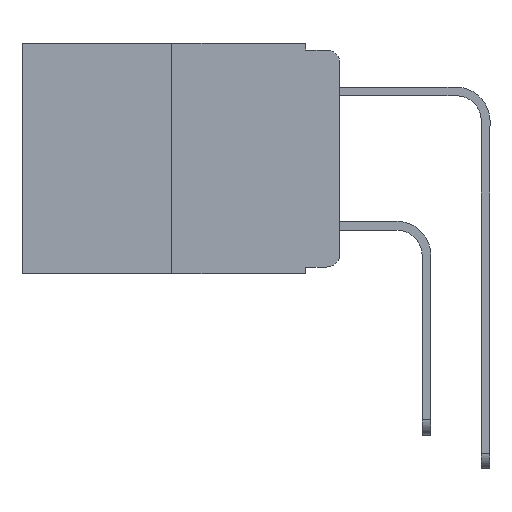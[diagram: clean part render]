
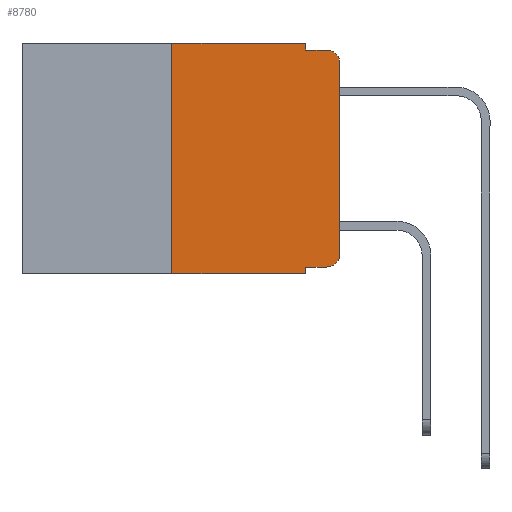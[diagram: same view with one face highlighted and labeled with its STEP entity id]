
A CAD part, left-side view. The second image highlights one B-rep face of the part: STEP entity #8780.
In plain terms, the highlighted planar face has unit normal (-1, 0, 0).
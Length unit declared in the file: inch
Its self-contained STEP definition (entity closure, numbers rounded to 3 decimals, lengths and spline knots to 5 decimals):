
#59 = VERTEX_POINT ( 'NONE', #3711 ) ;
#158 = VECTOR ( 'NONE', #4470, 39.37008 ) ;
#255 = DIRECTION ( 'NONE',  ( 0., 0., -1. ) ) ;
#367 = DIRECTION ( 'NONE',  ( 0., 0., -1. ) ) ;
#1039 = CARTESIAN_POINT ( 'NONE',  ( 0., 0.051, -0.01 ) ) ;
#1134 = LINE ( 'NONE', #12113, #1515 ) ;
#1308 = LINE ( 'NONE', #9074, #10703 ) ;
#1515 = VECTOR ( 'NONE', #367, 39.37008 ) ;
#1615 = LINE ( 'NONE', #4549, #13292 ) ;
#1960 = DIRECTION ( 'NONE',  ( 0., 0., 1. ) ) ;
#2012 = DIRECTION ( 'NONE',  ( -1., 0., 0. ) ) ;
#2083 = VERTEX_POINT ( 'NONE', #13262 ) ;
#2281 = DIRECTION ( 'NONE',  ( 0., -1., 0. ) ) ;
#2284 = LINE ( 'NONE', #9233, #8231 ) ;
#2569 = ORIENTED_EDGE ( 'NONE', *, *, #5013, .T. ) ;
#2573 = CARTESIAN_POINT ( 'NONE',  ( 0., 0.473, 0. ) ) ;
#3114 = ORIENTED_EDGE ( 'NONE', *, *, #7269, .F. ) ;
#3270 = VECTOR ( 'NONE', #5483, 39.37008 ) ;
#3467 = VECTOR ( 'NONE', #14346, 39.37008 ) ;
#3666 = ORIENTED_EDGE ( 'NONE', *, *, #6000, .F. ) ;
#3711 = CARTESIAN_POINT ( 'NONE',  ( 0., 0.25, -0.343 ) ) ;
#3911 = AXIS2_PLACEMENT_3D ( 'NONE', #9136, #2012, #10263 ) ;
#4214 = ORIENTED_EDGE ( 'NONE', *, *, #4797, .F. ) ;
#4291 = CARTESIAN_POINT ( 'NONE',  ( 0., 0.25, 0. ) ) ;
#4322 = CARTESIAN_POINT ( 'NONE',  ( 0., 0.02, -0.03 ) ) ;
#4470 = DIRECTION ( 'NONE',  ( 0., -1., 0. ) ) ;
#4549 = CARTESIAN_POINT ( 'NONE',  ( 0., 0.051, -0.333 ) ) ;
#4797 = EDGE_CURVE ( 'NONE', #13849, #8151, #1134, .T. ) ;
#4871 = CARTESIAN_POINT ( 'NONE',  ( 0., 0., -0.03 ) ) ;
#4902 = PLANE ( 'NONE',  #8077 ) ;
#5013 = EDGE_CURVE ( 'NONE', #2083, #12162, #1308, .T. ) ;
#5483 = DIRECTION ( 'NONE',  ( 0., 0., 1. ) ) ;
#5524 = DIRECTION ( 'NONE',  ( 0., 0., -1. ) ) ;
#6000 = EDGE_CURVE ( 'NONE', #6590, #13849, #9615, .T. ) ;
#6093 = LINE ( 'NONE', #12098, #3467 ) ;
#6144 = CARTESIAN_POINT ( 'NONE',  ( 0., 0.02, -0.01 ) ) ;
#6302 = ORIENTED_EDGE ( 'NONE', *, *, #8257, .T. ) ;
#6590 = VERTEX_POINT ( 'NONE', #6793 ) ;
#6793 = CARTESIAN_POINT ( 'NONE',  ( 0., 0.25, 0. ) ) ;
#6828 = EDGE_LOOP ( 'NONE', ( #2569, #6302, #3114, #4214, #3666, #13722, #14591, #10012, #12701, #13752 ) ) ;
#7088 = CARTESIAN_POINT ( 'NONE',  ( 0., 0.051, -0.333 ) ) ;
#7269 = EDGE_CURVE ( 'NONE', #8151, #12727, #9402, .T. ) ;
#7300 = EDGE_CURVE ( 'NONE', #7944, #7658, #1615, .T. ) ;
#7374 = DIRECTION ( 'NONE',  ( 1., 0., 0. ) ) ;
#7658 = VERTEX_POINT ( 'NONE', #10017 ) ;
#7944 = VERTEX_POINT ( 'NONE', #7088 ) ;
#8077 = AXIS2_PLACEMENT_3D ( 'NONE', #2573, #7374, #255 ) ;
#8148 = DIRECTION ( 'NONE',  ( 0., -1., 0. ) ) ;
#8151 = VERTEX_POINT ( 'NONE', #13424 ) ;
#8231 = VECTOR ( 'NONE', #10375, 39.37008 ) ;
#8257 = EDGE_CURVE ( 'NONE', #12162, #12727, #12726, .T. ) ;
#8293 = VECTOR ( 'NONE', #8148, 39.37008 ) ;
#8314 = VERTEX_POINT ( 'NONE', #9262 ) ;
#8780 = ADVANCED_FACE ( 'NONE', ( #14953 ), #4902, .F. ) ;
#9074 = CARTESIAN_POINT ( 'NONE',  ( 0., 0., 0. ) ) ;
#9136 = CARTESIAN_POINT ( 'NONE',  ( 0., 0.02, -0.313 ) ) ;
#9233 = CARTESIAN_POINT ( 'NONE',  ( 0., 0.051, 0. ) ) ;
#9262 = CARTESIAN_POINT ( 'NONE',  ( 0., 0.051, -0.343 ) ) ;
#9402 = LINE ( 'NONE', #1039, #8293 ) ;
#9615 = LINE ( 'NONE', #12675, #158 ) ;
#9961 = LINE ( 'NONE', #4291, #3270 ) ;
#10012 = ORIENTED_EDGE ( 'NONE', *, *, #14377, .F. ) ;
#10017 = CARTESIAN_POINT ( 'NONE',  ( 0., 0.02, -0.333 ) ) ;
#10263 = DIRECTION ( 'NONE',  ( 0., 0., -1. ) ) ;
#10375 = DIRECTION ( 'NONE',  ( 0., 0., -1. ) ) ;
#10629 = CARTESIAN_POINT ( 'NONE',  ( 0., 0.051, 0. ) ) ;
#10703 = VECTOR ( 'NONE', #1960, 39.37008 ) ;
#10749 = EDGE_CURVE ( 'NONE', #59, #8314, #6093, .T. ) ;
#10851 = EDGE_CURVE ( 'NONE', #59, #6590, #9961, .T. ) ;
#12098 = CARTESIAN_POINT ( 'NONE',  ( 0., 0.473, -0.343 ) ) ;
#12113 = CARTESIAN_POINT ( 'NONE',  ( 0., 0.051, 0. ) ) ;
#12162 = VERTEX_POINT ( 'NONE', #4871 ) ;
#12496 = AXIS2_PLACEMENT_3D ( 'NONE', #4322, #12538, #5524 ) ;
#12538 = DIRECTION ( 'NONE',  ( -1., 0., 0. ) ) ;
#12675 = CARTESIAN_POINT ( 'NONE',  ( 0., 0.473, 0. ) ) ;
#12701 = ORIENTED_EDGE ( 'NONE', *, *, #7300, .T. ) ;
#12726 = CIRCLE ( 'NONE', #12496, 0.02 ) ;
#12727 = VERTEX_POINT ( 'NONE', #6144 ) ;
#13262 = CARTESIAN_POINT ( 'NONE',  ( 0., 0., -0.313 ) ) ;
#13292 = VECTOR ( 'NONE', #2281, 39.37008 ) ;
#13424 = CARTESIAN_POINT ( 'NONE',  ( 0., 0.051, -0.01 ) ) ;
#13722 = ORIENTED_EDGE ( 'NONE', *, *, #10851, .F. ) ;
#13752 = ORIENTED_EDGE ( 'NONE', *, *, #14328, .T. ) ;
#13849 = VERTEX_POINT ( 'NONE', #10629 ) ;
#14328 = EDGE_CURVE ( 'NONE', #7658, #2083, #14962, .T. ) ;
#14346 = DIRECTION ( 'NONE',  ( 0., -1., 0. ) ) ;
#14377 = EDGE_CURVE ( 'NONE', #7944, #8314, #2284, .T. ) ;
#14591 = ORIENTED_EDGE ( 'NONE', *, *, #10749, .T. ) ;
#14953 = FACE_OUTER_BOUND ( 'NONE', #6828, .T. ) ;
#14962 = CIRCLE ( 'NONE', #3911, 0.02 ) ;
